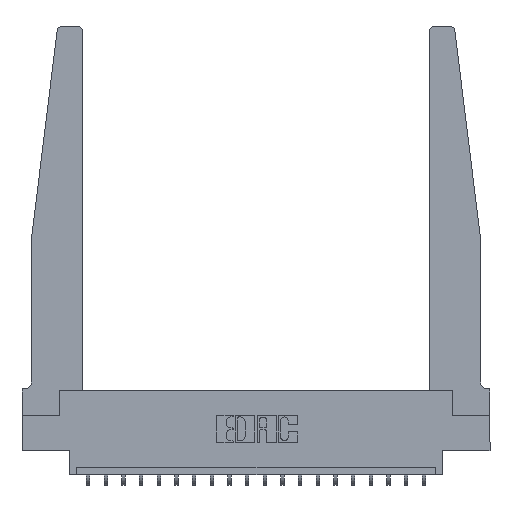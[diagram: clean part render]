
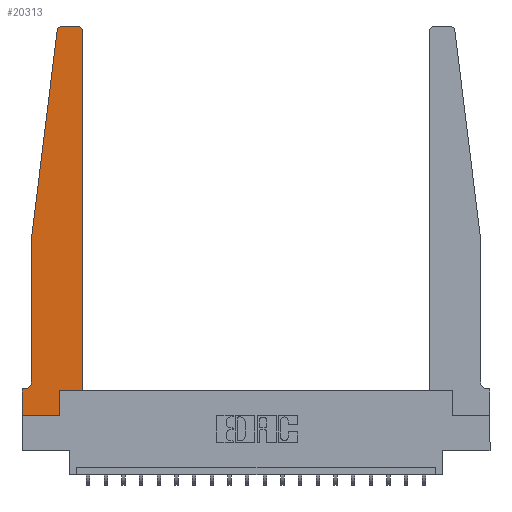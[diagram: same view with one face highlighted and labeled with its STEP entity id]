
A CAD part, top view. The second image highlights one B-rep face of the part: STEP entity #20313.
In plain terms, the highlighted planar face has unit normal (0, 0, 1).
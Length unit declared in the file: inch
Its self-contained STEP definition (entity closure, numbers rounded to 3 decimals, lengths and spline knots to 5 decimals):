
#287 = CARTESIAN_POINT ( 'NONE',  ( 0.065, 1.25, 0.37 ) ) ;
#387 = EDGE_CURVE ( 'NONE', #4644, #5684, #9122, .T. ) ;
#601 = DIRECTION ( 'NONE',  ( 1., 0., 0. ) ) ;
#869 = VERTEX_POINT ( 'NONE', #19886 ) ;
#1018 = ORIENTED_EDGE ( 'NONE', *, *, #13488, .T. ) ;
#1095 = CARTESIAN_POINT ( 'NONE',  ( 0.425, 2.72, 0.37 ) ) ;
#1530 = ORIENTED_EDGE ( 'NONE', *, *, #18159, .T. ) ;
#1649 = CARTESIAN_POINT ( 'NONE',  ( 0.25, 2.75, 0.37 ) ) ;
#1680 = VECTOR ( 'NONE', #7502, 39.37008 ) ;
#2285 = CARTESIAN_POINT ( 'NONE',  ( 0., 0.1875, 0.37 ) ) ;
#2322 = CARTESIAN_POINT ( 'NONE',  ( 0.065, 0.2375, 0.37 ) ) ;
#2429 = EDGE_CURVE ( 'NONE', #869, #15584, #3043, .T. ) ;
#3031 = ORIENTED_EDGE ( 'NONE', *, *, #16720, .T. ) ;
#3043 = LINE ( 'NONE', #8756, #19744 ) ;
#3464 = CARTESIAN_POINT ( 'NONE',  ( 0.2605, 0.18, 0.37 ) ) ;
#3663 = DIRECTION ( 'NONE',  ( 0., 0., 1. ) ) ;
#3813 = LINE ( 'NONE', #1649, #15837 ) ;
#3821 = VECTOR ( 'NONE', #10279, 39.37008 ) ;
#4049 = CARTESIAN_POINT ( 'NONE',  ( 0., 0., 0.37 ) ) ;
#4152 = CARTESIAN_POINT ( 'NONE',  ( 0.065, 0.1875, 0.37 ) ) ;
#4172 = FACE_OUTER_BOUND ( 'NONE', #15416, .T. ) ;
#4191 = LINE ( 'NONE', #13344, #12592 ) ;
#4644 = VERTEX_POINT ( 'NONE', #2285 ) ;
#4964 = DIRECTION ( 'NONE',  ( 1., 0., 0. ) ) ;
#5573 = DIRECTION ( 'NONE',  ( -0.122, -0.992, 0. ) ) ;
#5610 = EDGE_CURVE ( 'NONE', #6921, #7780, #7608, .T. ) ;
#5622 = CIRCLE ( 'NONE', #12210, 0.03 ) ;
#5671 = AXIS2_PLACEMENT_3D ( 'NONE', #12839, #14420, #4964 ) ;
#5684 = VERTEX_POINT ( 'NONE', #14537 ) ;
#5692 = LINE ( 'NONE', #18826, #18210 ) ;
#5723 = EDGE_CURVE ( 'NONE', #12686, #869, #5622, .T. ) ;
#5881 = AXIS2_PLACEMENT_3D ( 'NONE', #8159, #19095, #9726 ) ;
#6236 = ORIENTED_EDGE ( 'NONE', *, *, #387, .T. ) ;
#6921 = VERTEX_POINT ( 'NONE', #2322 ) ;
#7011 = DIRECTION ( 'NONE',  ( 0., 1., 0. ) ) ;
#7502 = DIRECTION ( 'NONE',  ( 0., -1., 0. ) ) ;
#7608 = CIRCLE ( 'NONE', #5881, 0.05 ) ;
#7728 = ORIENTED_EDGE ( 'NONE', *, *, #9363, .T. ) ;
#7780 = VERTEX_POINT ( 'NONE', #18435 ) ;
#7975 = ORIENTED_EDGE ( 'NONE', *, *, #5723, .T. ) ;
#8035 = LINE ( 'NONE', #16491, #3821 ) ;
#8159 = CARTESIAN_POINT ( 'NONE',  ( 0.015, 0.2375, 0.37 ) ) ;
#8171 = EDGE_CURVE ( 'NONE', #20053, #15801, #17323, .T. ) ;
#8256 = EDGE_CURVE ( 'NONE', #5684, #12813, #8035, .T. ) ;
#8756 = CARTESIAN_POINT ( 'NONE',  ( 0.065, 1.25, 0.37 ) ) ;
#9096 = LINE ( 'NONE', #13354, #12777 ) ;
#9122 = LINE ( 'NONE', #4049, #1680 ) ;
#9363 = EDGE_CURVE ( 'NONE', #11675, #20053, #9096, .T. ) ;
#9449 = ORIENTED_EDGE ( 'NONE', *, *, #5610, .T. ) ;
#9464 = DIRECTION ( 'NONE',  ( 0., -1., 0. ) ) ;
#9726 = DIRECTION ( 'NONE',  ( -1., 0., 0. ) ) ;
#10084 = DIRECTION ( 'NONE',  ( 0., 0., 1. ) ) ;
#10138 = AXIS2_PLACEMENT_3D ( 'NONE', #19453, #10084, #601 ) ;
#10279 = DIRECTION ( 'NONE',  ( 1., 0., 0. ) ) ;
#11245 = EDGE_CURVE ( 'NONE', #15801, #12686, #3813, .T. ) ;
#11251 = PLANE ( 'NONE',  #5671 ) ;
#11411 = ORIENTED_EDGE ( 'NONE', *, *, #19849, .T. ) ;
#11675 = VERTEX_POINT ( 'NONE', #13792 ) ;
#12210 = AXIS2_PLACEMENT_3D ( 'NONE', #13087, #3663, #14671 ) ;
#12407 = LINE ( 'NONE', #4152, #16056 ) ;
#12592 = VECTOR ( 'NONE', #17955, 39.37008 ) ;
#12686 = VERTEX_POINT ( 'NONE', #15115 ) ;
#12777 = VECTOR ( 'NONE', #7011, 39.37008 ) ;
#12813 = VERTEX_POINT ( 'NONE', #20137 ) ;
#12839 = CARTESIAN_POINT ( 'NONE',  ( 0., 0.1875, 0.37 ) ) ;
#13087 = CARTESIAN_POINT ( 'NONE',  ( 0.27653, 2.72, 0.37 ) ) ;
#13344 = CARTESIAN_POINT ( 'NONE',  ( 0.425, 0.18, 0.37 ) ) ;
#13354 = CARTESIAN_POINT ( 'NONE',  ( 0.425, 0.18, 0.37 ) ) ;
#13422 = CARTESIAN_POINT ( 'NONE',  ( 0.2605, 0.18, 0.37 ) ) ;
#13460 = VECTOR ( 'NONE', #15999, 39.37008 ) ;
#13488 = EDGE_CURVE ( 'NONE', #15584, #6921, #5692, .T. ) ;
#13546 = CARTESIAN_POINT ( 'NONE',  ( 0.395, 2.75, 0.37 ) ) ;
#13792 = CARTESIAN_POINT ( 'NONE',  ( 0.425, 0.18, 0.37 ) ) ;
#14420 = DIRECTION ( 'NONE',  ( 0., 0., 1. ) ) ;
#14482 = VERTEX_POINT ( 'NONE', #13422 ) ;
#14537 = CARTESIAN_POINT ( 'NONE',  ( 0., 0., 0.37 ) ) ;
#14671 = DIRECTION ( 'NONE',  ( 1., 0., 0. ) ) ;
#15115 = CARTESIAN_POINT ( 'NONE',  ( 0.27653, 2.75, 0.37 ) ) ;
#15416 = EDGE_LOOP ( 'NONE', ( #19474, #7975, #16281, #1018, #9449, #1530, #6236, #18740, #3031, #11411, #7728, #16048 ) ) ;
#15584 = VERTEX_POINT ( 'NONE', #287 ) ;
#15801 = VERTEX_POINT ( 'NONE', #13546 ) ;
#15837 = VECTOR ( 'NONE', #18969, 39.37008 ) ;
#15999 = DIRECTION ( 'NONE',  ( 0., 1., 0. ) ) ;
#16048 = ORIENTED_EDGE ( 'NONE', *, *, #8171, .T. ) ;
#16056 = VECTOR ( 'NONE', #16715, 39.37008 ) ;
#16281 = ORIENTED_EDGE ( 'NONE', *, *, #2429, .T. ) ;
#16491 = CARTESIAN_POINT ( 'NONE',  ( 0., 0., 0.37 ) ) ;
#16715 = DIRECTION ( 'NONE',  ( -1., 0., 0. ) ) ;
#16720 = EDGE_CURVE ( 'NONE', #12813, #14482, #17575, .T. ) ;
#17323 = CIRCLE ( 'NONE', #10138, 0.03 ) ;
#17575 = LINE ( 'NONE', #3464, #13460 ) ;
#17955 = DIRECTION ( 'NONE',  ( 1., 0., 0. ) ) ;
#18159 = EDGE_CURVE ( 'NONE', #7780, #4644, #12407, .T. ) ;
#18210 = VECTOR ( 'NONE', #9464, 39.37008 ) ;
#18435 = CARTESIAN_POINT ( 'NONE',  ( 0.015, 0.1875, 0.37 ) ) ;
#18740 = ORIENTED_EDGE ( 'NONE', *, *, #8256, .T. ) ;
#18826 = CARTESIAN_POINT ( 'NONE',  ( 0.065, 1.25, 0.37 ) ) ;
#18969 = DIRECTION ( 'NONE',  ( -1., 0., 0. ) ) ;
#19095 = DIRECTION ( 'NONE',  ( 0., 0., -1. ) ) ;
#19453 = CARTESIAN_POINT ( 'NONE',  ( 0.395, 2.72, 0.37 ) ) ;
#19474 = ORIENTED_EDGE ( 'NONE', *, *, #11245, .T. ) ;
#19744 = VECTOR ( 'NONE', #5573, 39.37008 ) ;
#19849 = EDGE_CURVE ( 'NONE', #14482, #11675, #4191, .T. ) ;
#19886 = CARTESIAN_POINT ( 'NONE',  ( 0.24675, 2.72367, 0.37 ) ) ;
#20053 = VERTEX_POINT ( 'NONE', #1095 ) ;
#20137 = CARTESIAN_POINT ( 'NONE',  ( 0.2605, 0., 0.37 ) ) ;
#20313 = ADVANCED_FACE ( 'NONE', ( #4172 ), #11251, .T. ) ;
